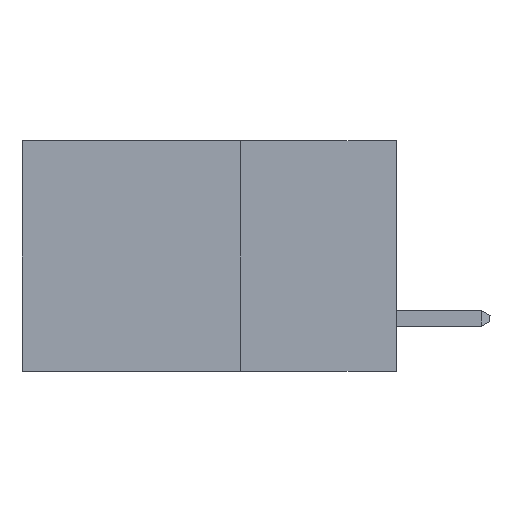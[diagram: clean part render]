
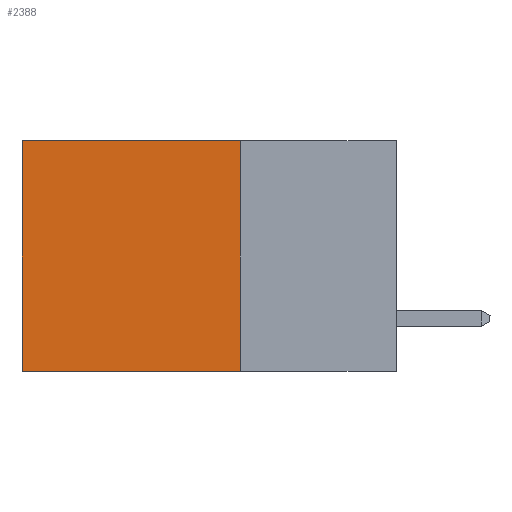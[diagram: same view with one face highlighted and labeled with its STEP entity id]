
A CAD part, left-side view. The second image highlights one B-rep face of the part: STEP entity #2388.
In plain terms, the highlighted planar face has unit normal (-1, 0, 0).
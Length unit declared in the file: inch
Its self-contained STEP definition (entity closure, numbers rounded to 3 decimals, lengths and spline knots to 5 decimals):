
#197 = EDGE_CURVE ( 'NONE', #6838, #7934, #16156, .T. ) ;
#1013 = CARTESIAN_POINT ( 'NONE',  ( 0.2615, 0.6, -0.37 ) ) ;
#1077 = VERTEX_POINT ( 'NONE', #8279 ) ;
#1397 = DIRECTION ( 'NONE',  ( 0., 0., -1. ) ) ;
#1876 = CARTESIAN_POINT ( 'NONE',  ( 0.2615, 0.25, 0. ) ) ;
#1970 = EDGE_CURVE ( 'NONE', #6838, #1077, #10744, .T. ) ;
#2388 = ADVANCED_FACE ( 'NONE', ( #5639 ), #16419, .F. ) ;
#2688 = VECTOR ( 'NONE', #13145, 39.37008 ) ;
#2924 = EDGE_CURVE ( 'NONE', #1077, #16440, #11207, .T. ) ;
#3332 = DIRECTION ( 'NONE',  ( 0., 1., 0. ) ) ;
#3540 = EDGE_LOOP ( 'NONE', ( #15604, #15189, #7032, #5714 ) ) ;
#4317 = CARTESIAN_POINT ( 'NONE',  ( 0.2615, 0.25, -0.37 ) ) ;
#5166 = EDGE_CURVE ( 'NONE', #7934, #16440, #14194, .T. ) ;
#5358 = DIRECTION ( 'NONE',  ( 0., 1., 0. ) ) ;
#5639 = FACE_OUTER_BOUND ( 'NONE', #3540, .T. ) ;
#5714 = ORIENTED_EDGE ( 'NONE', *, *, #197, .T. ) ;
#6838 = VERTEX_POINT ( 'NONE', #1876 ) ;
#7032 = ORIENTED_EDGE ( 'NONE', *, *, #1970, .F. ) ;
#7934 = VERTEX_POINT ( 'NONE', #16387 ) ;
#8279 = CARTESIAN_POINT ( 'NONE',  ( 0.2615, 0.25, -0.37 ) ) ;
#9566 = CARTESIAN_POINT ( 'NONE',  ( 0.2615, 0.25, 0. ) ) ;
#9648 = DIRECTION ( 'NONE',  ( 0., 0., -1. ) ) ;
#10744 = LINE ( 'NONE', #14909, #17085 ) ;
#11149 = AXIS2_PLACEMENT_3D ( 'NONE', #4317, #12353, #9648 ) ;
#11207 = LINE ( 'NONE', #16846, #14443 ) ;
#12353 = DIRECTION ( 'NONE',  ( 1., 0., 0. ) ) ;
#13145 = DIRECTION ( 'NONE',  ( 0., 0., -1. ) ) ;
#14194 = LINE ( 'NONE', #1013, #2688 ) ;
#14443 = VECTOR ( 'NONE', #3332, 39.37008 ) ;
#14909 = CARTESIAN_POINT ( 'NONE',  ( 0.2615, 0.25, -0.37 ) ) ;
#15189 = ORIENTED_EDGE ( 'NONE', *, *, #2924, .F. ) ;
#15604 = ORIENTED_EDGE ( 'NONE', *, *, #5166, .T. ) ;
#15917 = VECTOR ( 'NONE', #5358, 39.37008 ) ;
#16156 = LINE ( 'NONE', #9566, #15917 ) ;
#16387 = CARTESIAN_POINT ( 'NONE',  ( 0.2615, 0.6, 0. ) ) ;
#16419 = PLANE ( 'NONE',  #11149 ) ;
#16440 = VERTEX_POINT ( 'NONE', #16458 ) ;
#16458 = CARTESIAN_POINT ( 'NONE',  ( 0.2615, 0.6, -0.37 ) ) ;
#16846 = CARTESIAN_POINT ( 'NONE',  ( 0.2615, 0.25, -0.37 ) ) ;
#17085 = VECTOR ( 'NONE', #1397, 39.37008 ) ;
